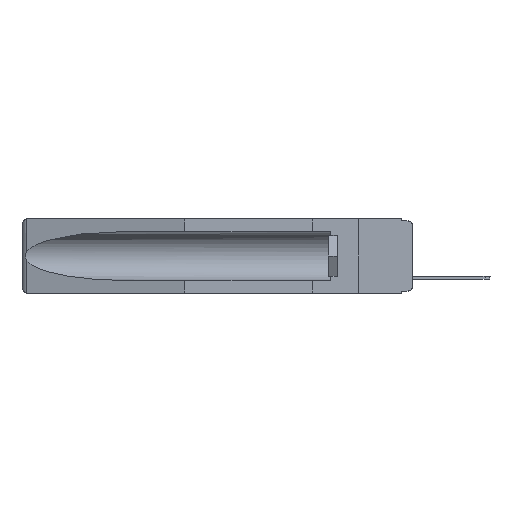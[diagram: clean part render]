
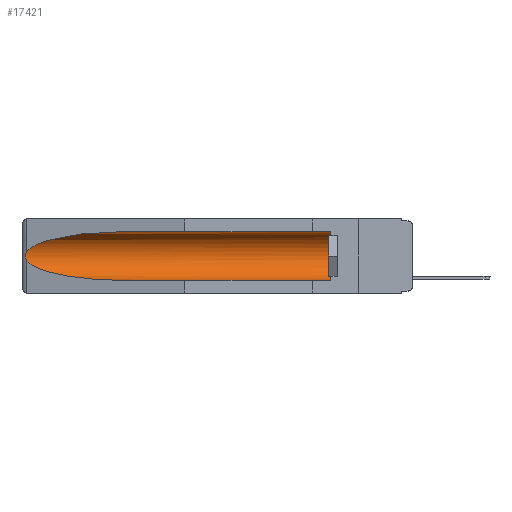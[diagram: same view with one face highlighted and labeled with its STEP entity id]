
A CAD part, left-side view. The second image highlights one B-rep face of the part: STEP entity #17421.
In plain terms, the highlighted cylindrical face has radius 2.857 mm (diameter 5.715 mm), a partial arc.
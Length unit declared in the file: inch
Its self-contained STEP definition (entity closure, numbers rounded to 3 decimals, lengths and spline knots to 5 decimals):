
#283 = CARTESIAN_POINT ( 'NONE',  ( 0.155, 0.126, -0.284 ) ) ;
#706 = VERTEX_POINT ( 'NONE', #17069 ) ;
#2164 = ORIENTED_EDGE ( 'NONE', *, *, #3865, .T. ) ;
#2821 = CARTESIAN_POINT ( 'NONE',  ( 0.26537, 1.52718, -0.19328 ) ) ;
#2837 = ORIENTED_EDGE ( 'NONE', *, *, #18227, .T. ) ;
#2888 = CARTESIAN_POINT ( 'NONE',  ( 0.155, 0.126, -0.059 ) ) ;
#3588 = EDGE_LOOP ( 'NONE', ( #2837, #2164, #20099, #13952, #4508, #11879 ) ) ;
#3680 = VERTEX_POINT ( 'NONE', #6040 ) ;
#3720 = EDGE_CURVE ( 'NONE', #18809, #18693, #4002, .T. ) ;
#3865 = EDGE_CURVE ( 'NONE', #3680, #20640, #7199, .T. ) ;
#4002 = CIRCLE ( 'NONE', #6804, 0.1125 ) ;
#4466 = CARTESIAN_POINT ( 'NONE',  ( 0.155, -0.30754, -0.284 ) ) ;
#4508 = ORIENTED_EDGE ( 'NONE', *, *, #3720, .T. ) ;
#4882 = CARTESIAN_POINT ( 'NONE',  ( 0.155, 1.07973, -0.059 ) ) ;
#5637 = VERTEX_POINT ( 'NONE', #11408 ) ;
#6040 = CARTESIAN_POINT ( 'NONE',  ( 0.26537, 1.52718, -0.14972 ) ) ;
#6075 = CARTESIAN_POINT ( 'NONE',  ( 0.26654, 1.53092, -0.15636 ) ) ;
#6258 = DIRECTION ( 'NONE',  ( 0., 0., 1. ) ) ;
#6411 = CARTESIAN_POINT ( 'NONE',  ( 0.26537, 1.52718, -0.14972 ) ) ;
#6580 = DIRECTION ( 'NONE',  ( 0., 0., 1. ) ) ;
#6804 = AXIS2_PLACEMENT_3D ( 'NONE', #9325, #21196, #6258 ) ;
#7138 = LINE ( 'NONE', #15319, #19238 ) ;
#7199 = B_SPLINE_CURVE_WITH_KNOTS ( 'NONE', 3,
 ( #14254, #7943, #6075, #17744, #21228, #19172, #12635, #9470, #8050, #12955 ),
 .UNSPECIFIED., .F., .F.,
 ( 4, 2, 2, 2, 4 ),
 ( 0., 0.00029, 0.00058, 0.00087, 0.00117 ),
 .UNSPECIFIED. ) ;
#7450 =( BOUNDED_CURVE ( )  B_SPLINE_CURVE ( 3, ( #4882, #11548, #16553, #6411 ),
 .UNSPECIFIED., .F., .F. ) 
 B_SPLINE_CURVE_WITH_KNOTS ( ( 4, 4 ),
 ( 4.71239, 6.08839 ),
 .UNSPECIFIED. ) 
 CURVE ( )  GEOMETRIC_REPRESENTATION_ITEM ( )  RATIONAL_B_SPLINE_CURVE ( ( 1., 0.848, 0.848, 1. ) ) 
 REPRESENTATION_ITEM ( '' )  );
#7943 = CARTESIAN_POINT ( 'NONE',  ( 0.26597, 1.52961, -0.15275 ) ) ;
#8050 = CARTESIAN_POINT ( 'NONE',  ( 0.26597, 1.5296, -0.19026 ) ) ;
#8228 = CARTESIAN_POINT ( 'NONE',  ( 0.155, -0.30754, -0.1715 ) ) ;
#9325 = CARTESIAN_POINT ( 'NONE',  ( 0.155, 0.126, -0.1715 ) ) ;
#9470 = CARTESIAN_POINT ( 'NONE',  ( 0.26655, 1.53094, -0.18657 ) ) ;
#11408 = CARTESIAN_POINT ( 'NONE',  ( 0.155, 1.07973, -0.284 ) ) ;
#11548 = CARTESIAN_POINT ( 'NONE',  ( 0.21114, 1.30732, -0.059 ) ) ;
#11879 = ORIENTED_EDGE ( 'NONE', *, *, #12746, .T. ) ;
#12221 = CARTESIAN_POINT ( 'NONE',  ( 0.21114, 1.30732, -0.284 ) ) ;
#12635 = CARTESIAN_POINT ( 'NONE',  ( 0.2673, 1.53269, -0.17917 ) ) ;
#12746 = EDGE_CURVE ( 'NONE', #18693, #706, #7138, .T. ) ;
#12955 = CARTESIAN_POINT ( 'NONE',  ( 0.26537, 1.52718, -0.19328 ) ) ;
#13847 = CARTESIAN_POINT ( 'NONE',  ( 0.25451, 1.48313, -0.24835 ) ) ;
#13952 = ORIENTED_EDGE ( 'NONE', *, *, #16583, .F. ) ;
#14254 = CARTESIAN_POINT ( 'NONE',  ( 0.26537, 1.52718, -0.14972 ) ) ;
#14255 =( BOUNDED_CURVE ( )  B_SPLINE_CURVE ( 3, ( #20911, #13847, #12221, #16007 ),
 .UNSPECIFIED., .F., .F. ) 
 B_SPLINE_CURVE_WITH_KNOTS ( ( 4, 4 ),
 ( 0.1948, 1.5708 ),
 .UNSPECIFIED. ) 
 CURVE ( )  GEOMETRIC_REPRESENTATION_ITEM ( )  RATIONAL_B_SPLINE_CURVE ( ( 1., 0.848, 0.848, 1. ) ) 
 REPRESENTATION_ITEM ( '' )  );
#15319 = CARTESIAN_POINT ( 'NONE',  ( 0.155, -0.30754, -0.059 ) ) ;
#16007 = CARTESIAN_POINT ( 'NONE',  ( 0.155, 1.07973, -0.284 ) ) ;
#16251 = DIRECTION ( 'NONE',  ( 0., 1., 0. ) ) ;
#16553 = CARTESIAN_POINT ( 'NONE',  ( 0.25451, 1.48313, -0.09465 ) ) ;
#16583 = EDGE_CURVE ( 'NONE', #18809, #5637, #17891, .T. ) ;
#16834 = EDGE_CURVE ( 'NONE', #20640, #5637, #14255, .T. ) ;
#17069 = CARTESIAN_POINT ( 'NONE',  ( 0.155, 1.07973, -0.059 ) ) ;
#17421 = ADVANCED_FACE ( 'NONE', ( #19783 ), #19887, .F. ) ;
#17744 = CARTESIAN_POINT ( 'NONE',  ( 0.2673, 1.5327, -0.16383 ) ) ;
#17891 = LINE ( 'NONE', #4466, #18622 ) ;
#18227 = EDGE_CURVE ( 'NONE', #706, #3680, #7450, .T. ) ;
#18622 = VECTOR ( 'NONE', #16251, 39.37008 ) ;
#18693 = VERTEX_POINT ( 'NONE', #2888 ) ;
#18809 = VERTEX_POINT ( 'NONE', #283 ) ;
#19172 = CARTESIAN_POINT ( 'NONE',  ( 0.2675, 1.53308, -0.17534 ) ) ;
#19238 = VECTOR ( 'NONE', #20758, 39.37008 ) ;
#19783 = FACE_OUTER_BOUND ( 'NONE', #3588, .T. ) ;
#19887 = CYLINDRICAL_SURFACE ( 'NONE', #20030, 0.1125 ) ;
#20030 = AXIS2_PLACEMENT_3D ( 'NONE', #8228, #21523, #6580 ) ;
#20099 = ORIENTED_EDGE ( 'NONE', *, *, #16834, .T. ) ;
#20640 = VERTEX_POINT ( 'NONE', #2821 ) ;
#20758 = DIRECTION ( 'NONE',  ( 0., 1., 0. ) ) ;
#20911 = CARTESIAN_POINT ( 'NONE',  ( 0.26537, 1.52718, -0.19328 ) ) ;
#21196 = DIRECTION ( 'NONE',  ( 0., -1., 0. ) ) ;
#21228 = CARTESIAN_POINT ( 'NONE',  ( 0.2675, 1.53308, -0.16763 ) ) ;
#21523 = DIRECTION ( 'NONE',  ( 0., 1., 0. ) ) ;
